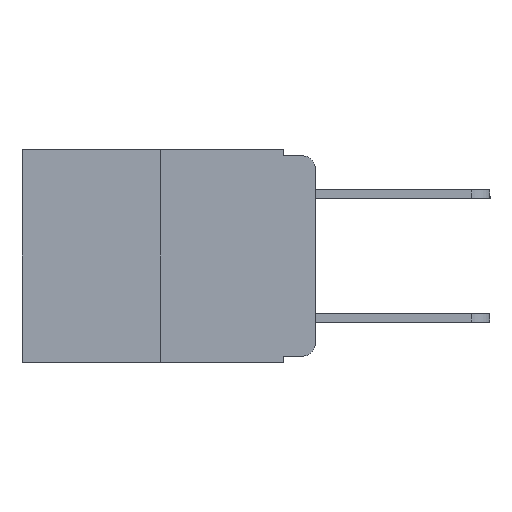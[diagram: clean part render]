
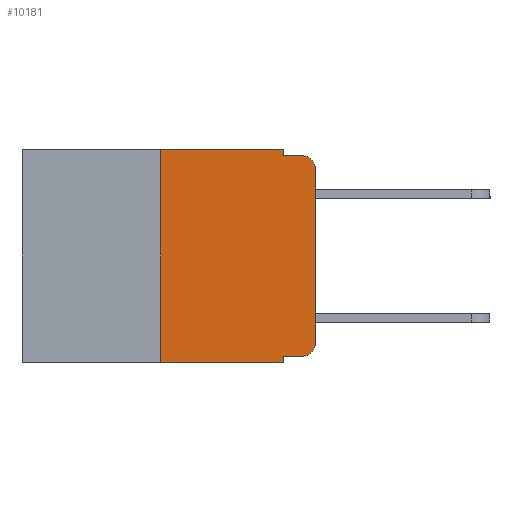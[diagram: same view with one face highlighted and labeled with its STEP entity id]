
A CAD part, left-side view. The second image highlights one B-rep face of the part: STEP entity #10181.
In plain terms, the highlighted planar face has unit normal (-1, 0, 0).
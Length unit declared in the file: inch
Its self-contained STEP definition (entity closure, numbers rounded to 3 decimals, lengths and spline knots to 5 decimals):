
#70 = ORIENTED_EDGE ( 'NONE', *, *, #925, .T. ) ;
#114 = CARTESIAN_POINT ( 'NONE',  ( 0., 0., 0. ) ) ;
#423 = EDGE_CURVE ( 'NONE', #1571, #7093, #2135, .T. ) ;
#791 = VERTEX_POINT ( 'NONE', #10484 ) ;
#915 = EDGE_CURVE ( 'NONE', #4857, #6509, #9682, .T. ) ;
#925 = EDGE_CURVE ( 'NONE', #7093, #6509, #9198, .T. ) ;
#992 = CARTESIAN_POINT ( 'NONE',  ( 0., 0.02, -0.333 ) ) ;
#1281 = CIRCLE ( 'NONE', #2895, 0.02 ) ;
#1469 = LINE ( 'NONE', #4119, #10285 ) ;
#1569 = EDGE_CURVE ( 'NONE', #791, #4857, #4156, .T. ) ;
#1571 = VERTEX_POINT ( 'NONE', #10320 ) ;
#1691 = LINE ( 'NONE', #3877, #10459 ) ;
#2038 = EDGE_CURVE ( 'NONE', #3074, #10236, #1691, .T. ) ;
#2135 = LINE ( 'NONE', #114, #10754 ) ;
#2138 = EDGE_CURVE ( 'NONE', #2756, #7555, #10987, .T. ) ;
#2159 = CARTESIAN_POINT ( 'NONE',  ( 0., 0.02, -0.01 ) ) ;
#2468 = VECTOR ( 'NONE', #9270, 39.37008 ) ;
#2578 = CARTESIAN_POINT ( 'NONE',  ( 0., 0.473, 0. ) ) ;
#2630 = DIRECTION ( 'NONE',  ( 0., 0., -1. ) ) ;
#2643 = DIRECTION ( 'NONE',  ( 1., 0., 0. ) ) ;
#2650 = ORIENTED_EDGE ( 'NONE', *, *, #423, .T. ) ;
#2756 = VERTEX_POINT ( 'NONE', #4451 ) ;
#2762 = PLANE ( 'NONE',  #10123 ) ;
#2895 = AXIS2_PLACEMENT_3D ( 'NONE', #7166, #7157, #7125 ) ;
#2998 = DIRECTION ( 'NONE',  ( 0., -1., 0. ) ) ;
#3025 = CARTESIAN_POINT ( 'NONE',  ( 0., 0.473, 0. ) ) ;
#3074 = VERTEX_POINT ( 'NONE', #4312 ) ;
#3379 = VERTEX_POINT ( 'NONE', #4026 ) ;
#3523 = ORIENTED_EDGE ( 'NONE', *, *, #915, .F. ) ;
#3724 = DIRECTION ( 'NONE',  ( 0., 0., 1. ) ) ;
#3877 = CARTESIAN_POINT ( 'NONE',  ( 0., 0.051, -0.333 ) ) ;
#3915 = DIRECTION ( 'NONE',  ( 0., -1., 0. ) ) ;
#4026 = CARTESIAN_POINT ( 'NONE',  ( 0., 0.051, -0.343 ) ) ;
#4119 = CARTESIAN_POINT ( 'NONE',  ( 0., 0.051, 0. ) ) ;
#4133 = ORIENTED_EDGE ( 'NONE', *, *, #9355, .F. ) ;
#4156 = LINE ( 'NONE', #9964, #6249 ) ;
#4161 = ORIENTED_EDGE ( 'NONE', *, *, #1569, .F. ) ;
#4312 = CARTESIAN_POINT ( 'NONE',  ( 0., 0.051, -0.333 ) ) ;
#4378 = ORIENTED_EDGE ( 'NONE', *, *, #2138, .F. ) ;
#4451 = CARTESIAN_POINT ( 'NONE',  ( 0., 0.25, -0.343 ) ) ;
#4476 = ORIENTED_EDGE ( 'NONE', *, *, #8586, .T. ) ;
#4707 = EDGE_LOOP ( 'NONE', ( #2650, #70, #3523, #4161, #4133, #4378, #4476, #8071, #6886, #6325 ) ) ;
#4857 = VERTEX_POINT ( 'NONE', #10565 ) ;
#5033 = VECTOR ( 'NONE', #6632, 39.37008 ) ;
#5305 = FACE_OUTER_BOUND ( 'NONE', #4707, .T. ) ;
#5611 = DIRECTION ( 'NONE',  ( 0., 0., -1. ) ) ;
#6221 = CARTESIAN_POINT ( 'NONE',  ( 0., 0., -0.03 ) ) ;
#6249 = VECTOR ( 'NONE', #10950, 39.37008 ) ;
#6325 = ORIENTED_EDGE ( 'NONE', *, *, #8865, .T. ) ;
#6419 = CARTESIAN_POINT ( 'NONE',  ( 0., 0.051, -0.01 ) ) ;
#6509 = VERTEX_POINT ( 'NONE', #2159 ) ;
#6632 = DIRECTION ( 'NONE',  ( 0., -1., 0. ) ) ;
#6686 = LINE ( 'NONE', #3025, #10605 ) ;
#6886 = ORIENTED_EDGE ( 'NONE', *, *, #2038, .T. ) ;
#6910 = CARTESIAN_POINT ( 'NONE',  ( 0., 0.25, 0. ) ) ;
#7070 = CARTESIAN_POINT ( 'NONE',  ( 0., 0.02, -0.03 ) ) ;
#7093 = VERTEX_POINT ( 'NONE', #6221 ) ;
#7125 = DIRECTION ( 'NONE',  ( 0., 0., -1. ) ) ;
#7157 = DIRECTION ( 'NONE',  ( -1., 0., 0. ) ) ;
#7166 = CARTESIAN_POINT ( 'NONE',  ( 0., 0.02, -0.313 ) ) ;
#7328 = AXIS2_PLACEMENT_3D ( 'NONE', #7070, #7714, #5611 ) ;
#7356 = EDGE_CURVE ( 'NONE', #3074, #3379, #1469, .T. ) ;
#7555 = VERTEX_POINT ( 'NONE', #6910 ) ;
#7714 = DIRECTION ( 'NONE',  ( -1., 0., 0. ) ) ;
#8071 = ORIENTED_EDGE ( 'NONE', *, *, #7356, .F. ) ;
#8142 = DIRECTION ( 'NONE',  ( 0., -1., 0. ) ) ;
#8586 = EDGE_CURVE ( 'NONE', #2756, #3379, #10728, .T. ) ;
#8865 = EDGE_CURVE ( 'NONE', #10236, #1571, #1281, .T. ) ;
#9167 = CARTESIAN_POINT ( 'NONE',  ( 0., 0.25, 0. ) ) ;
#9195 = CARTESIAN_POINT ( 'NONE',  ( 0., 0.473, -0.343 ) ) ;
#9198 = CIRCLE ( 'NONE', #7328, 0.02 ) ;
#9270 = DIRECTION ( 'NONE',  ( 0., 0., 1. ) ) ;
#9355 = EDGE_CURVE ( 'NONE', #7555, #791, #6686, .T. ) ;
#9682 = LINE ( 'NONE', #6419, #5033 ) ;
#9818 = DIRECTION ( 'NONE',  ( 0., 0., -1. ) ) ;
#9964 = CARTESIAN_POINT ( 'NONE',  ( 0., 0.051, 0. ) ) ;
#10123 = AXIS2_PLACEMENT_3D ( 'NONE', #2578, #2643, #2630 ) ;
#10181 = ADVANCED_FACE ( 'NONE', ( #5305 ), #2762, .F. ) ;
#10236 = VERTEX_POINT ( 'NONE', #992 ) ;
#10285 = VECTOR ( 'NONE', #9818, 39.37008 ) ;
#10320 = CARTESIAN_POINT ( 'NONE',  ( 0., 0., -0.313 ) ) ;
#10459 = VECTOR ( 'NONE', #3915, 39.37008 ) ;
#10484 = CARTESIAN_POINT ( 'NONE',  ( 0., 0.051, 0. ) ) ;
#10504 = VECTOR ( 'NONE', #8142, 39.37008 ) ;
#10565 = CARTESIAN_POINT ( 'NONE',  ( 0., 0.051, -0.01 ) ) ;
#10605 = VECTOR ( 'NONE', #2998, 39.37008 ) ;
#10728 = LINE ( 'NONE', #9195, #10504 ) ;
#10754 = VECTOR ( 'NONE', #3724, 39.37008 ) ;
#10950 = DIRECTION ( 'NONE',  ( 0., 0., -1. ) ) ;
#10987 = LINE ( 'NONE', #9167, #2468 ) ;
